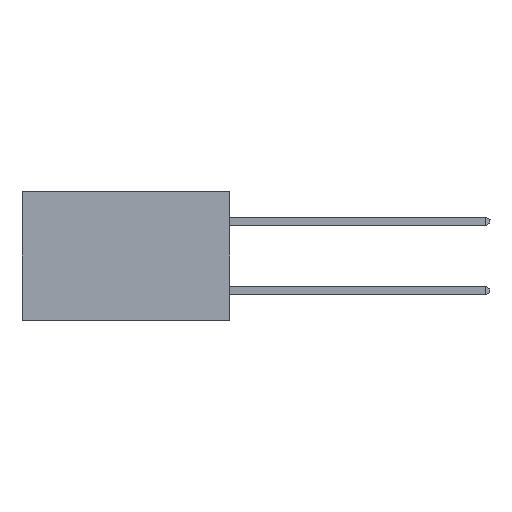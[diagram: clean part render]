
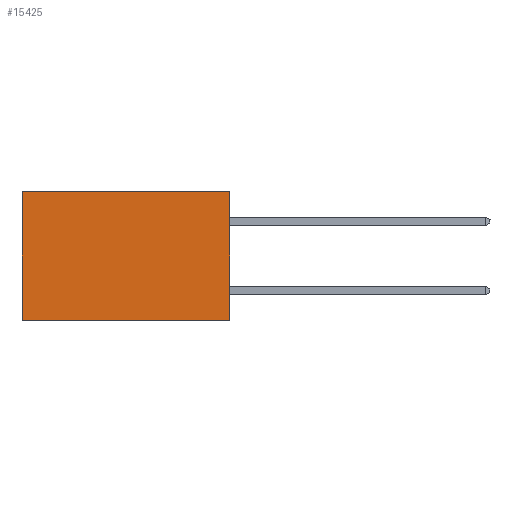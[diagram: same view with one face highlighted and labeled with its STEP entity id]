
A CAD part, left-side view. The second image highlights one B-rep face of the part: STEP entity #15425.
In plain terms, the highlighted planar face has unit normal (-1, 0, 0).
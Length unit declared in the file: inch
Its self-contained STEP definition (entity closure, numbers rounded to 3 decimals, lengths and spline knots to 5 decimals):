
#103 = VERTEX_POINT ( 'NONE', #12703 ) ;
#1234 = DIRECTION ( 'NONE',  ( 0., 0., -1. ) ) ;
#2774 = VECTOR ( 'NONE', #17000, 39.37008 ) ;
#2914 = DIRECTION ( 'NONE',  ( 0., 0., -1. ) ) ;
#3614 = CARTESIAN_POINT ( 'NONE',  ( 0.298, 0., -0.37 ) ) ;
#3971 = CARTESIAN_POINT ( 'NONE',  ( 0.298, 0., 0. ) ) ;
#4463 = VECTOR ( 'NONE', #16658, 39.37008 ) ;
#5390 = LINE ( 'NONE', #20881, #14095 ) ;
#5561 = DIRECTION ( 'NONE',  ( 1., 0., 0. ) ) ;
#6924 = EDGE_CURVE ( 'NONE', #7456, #9611, #10143, .T. ) ;
#7456 = VERTEX_POINT ( 'NONE', #8926 ) ;
#8030 = EDGE_CURVE ( 'NONE', #9611, #103, #19540, .T. ) ;
#8117 = DIRECTION ( 'NONE',  ( 0., 0., -1. ) ) ;
#8295 = ORIENTED_EDGE ( 'NONE', *, *, #18868, .F. ) ;
#8926 = CARTESIAN_POINT ( 'NONE',  ( 0.298, 0., 0. ) ) ;
#9611 = VERTEX_POINT ( 'NONE', #11397 ) ;
#10143 = LINE ( 'NONE', #3971, #4463 ) ;
#11373 = VERTEX_POINT ( 'NONE', #3614 ) ;
#11397 = CARTESIAN_POINT ( 'NONE',  ( 0.298, 0.6, 0. ) ) ;
#11605 = AXIS2_PLACEMENT_3D ( 'NONE', #22724, #5561, #1234 ) ;
#11704 = EDGE_LOOP ( 'NONE', ( #27335, #24203, #8295, #22100 ) ) ;
#12435 = VECTOR ( 'NONE', #2914, 39.37008 ) ;
#12703 = CARTESIAN_POINT ( 'NONE',  ( 0.298, 0.6, -0.37 ) ) ;
#14095 = VECTOR ( 'NONE', #8117, 39.37008 ) ;
#14286 = PLANE ( 'NONE',  #11605 ) ;
#14815 = CARTESIAN_POINT ( 'NONE',  ( 0.298, 0., -0.37 ) ) ;
#15425 = ADVANCED_FACE ( 'NONE', ( #16922 ), #14286, .F. ) ;
#16658 = DIRECTION ( 'NONE',  ( 0., 1., 0. ) ) ;
#16922 = FACE_OUTER_BOUND ( 'NONE', #11704, .T. ) ;
#17000 = DIRECTION ( 'NONE',  ( 0., 1., 0. ) ) ;
#17123 = EDGE_CURVE ( 'NONE', #11373, #103, #26624, .T. ) ;
#18868 = EDGE_CURVE ( 'NONE', #7456, #11373, #5390, .T. ) ;
#19540 = LINE ( 'NONE', #20131, #12435 ) ;
#20131 = CARTESIAN_POINT ( 'NONE',  ( 0.298, 0.6, 0. ) ) ;
#20881 = CARTESIAN_POINT ( 'NONE',  ( 0.298, 0., 0. ) ) ;
#22100 = ORIENTED_EDGE ( 'NONE', *, *, #6924, .T. ) ;
#22724 = CARTESIAN_POINT ( 'NONE',  ( 0.298, 0., 0. ) ) ;
#24203 = ORIENTED_EDGE ( 'NONE', *, *, #17123, .F. ) ;
#26624 = LINE ( 'NONE', #14815, #2774 ) ;
#27335 = ORIENTED_EDGE ( 'NONE', *, *, #8030, .T. ) ;
